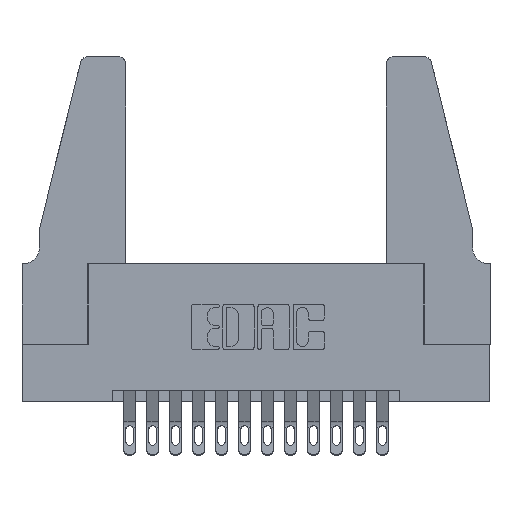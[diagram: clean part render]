
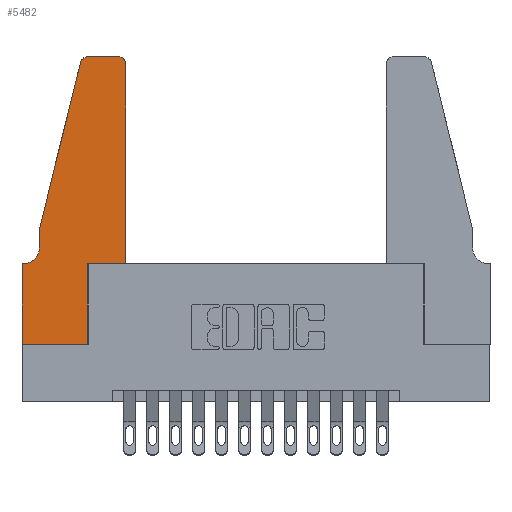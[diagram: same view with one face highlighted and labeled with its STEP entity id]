
A CAD part, top view. The second image highlights one B-rep face of the part: STEP entity #5482.
In plain terms, the highlighted planar face has unit normal (0, 0, 1).
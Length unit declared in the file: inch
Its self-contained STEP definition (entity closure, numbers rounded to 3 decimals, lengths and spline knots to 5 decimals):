
#66 = DIRECTION ( 'NONE',  ( 1., 0., 0. ) ) ;
#68 = EDGE_CURVE ( 'NONE', #10396, #11256, #2403, .T. ) ;
#447 = ORIENTED_EDGE ( 'NONE', *, *, #14626, .T. ) ;
#499 = DIRECTION ( 'NONE',  ( 1., 0., 0. ) ) ;
#636 = ORIENTED_EDGE ( 'NONE', *, *, #12247, .T. ) ;
#896 = DIRECTION ( 'NONE',  ( -1., 0., 0. ) ) ;
#1134 = VECTOR ( 'NONE', #2649, 39.37008 ) ;
#1259 = CARTESIAN_POINT ( 'NONE',  ( 0.284, 1.25, 0.37 ) ) ;
#1602 = CIRCLE ( 'NONE', #11623, 0.03 ) ;
#1690 = CARTESIAN_POINT ( 'NONE',  ( 0., 0., 0.37 ) ) ;
#1695 = DIRECTION ( 'NONE',  ( 0., 0., -1. ) ) ;
#1731 = ORIENTED_EDGE ( 'NONE', *, *, #14459, .T. ) ;
#1764 = CARTESIAN_POINT ( 'NONE',  ( 0., 0., 0.37 ) ) ;
#2403 = CIRCLE ( 'NONE', #11865, 0.07 ) ;
#2626 = LINE ( 'NONE', #1690, #5271 ) ;
#2649 = DIRECTION ( 'NONE',  ( 0., -1., 0. ) ) ;
#2809 = VECTOR ( 'NONE', #12594, 39.37008 ) ;
#2885 = CARTESIAN_POINT ( 'NONE',  ( 0.0055, 0.42, 0.37 ) ) ;
#2941 = DIRECTION ( 'NONE',  ( 0., 0., 1. ) ) ;
#3210 = DIRECTION ( 'NONE',  ( 1., 0., 0. ) ) ;
#3845 = VECTOR ( 'NONE', #13392, 39.37008 ) ;
#4041 = LINE ( 'NONE', #14674, #3845 ) ;
#4097 = EDGE_CURVE ( 'NONE', #15137, #5922, #13738, .T. ) ;
#4309 = VERTEX_POINT ( 'NONE', #12891 ) ;
#4357 = ORIENTED_EDGE ( 'NONE', *, *, #68, .T. ) ;
#4721 = CARTESIAN_POINT ( 'NONE',  ( 0.0755, 0.5, 0.37 ) ) ;
#4800 = FACE_OUTER_BOUND ( 'NONE', #14989, .T. ) ;
#4968 = ORIENTED_EDGE ( 'NONE', *, *, #10541, .T. ) ;
#5118 = DIRECTION ( 'NONE',  ( 1., 0., 0. ) ) ;
#5167 = CARTESIAN_POINT ( 'NONE',  ( 0.4505, 0.35, 0.37 ) ) ;
#5209 = ORIENTED_EDGE ( 'NONE', *, *, #5463, .T. ) ;
#5271 = VECTOR ( 'NONE', #499, 39.37008 ) ;
#5394 = DIRECTION ( 'NONE',  ( 0., 0., 1. ) ) ;
#5406 = VECTOR ( 'NONE', #5118, 39.37008 ) ;
#5433 = VERTEX_POINT ( 'NONE', #14991 ) ;
#5463 = EDGE_CURVE ( 'NONE', #6011, #7931, #13509, .T. ) ;
#5482 = ADVANCED_FACE ( 'NONE', ( #4800 ), #13869, .T. ) ;
#5524 = VERTEX_POINT ( 'NONE', #1764 ) ;
#5792 = EDGE_CURVE ( 'NONE', #5933, #8290, #8317, .T. ) ;
#5863 = LINE ( 'NONE', #11382, #2809 ) ;
#5922 = VERTEX_POINT ( 'NONE', #4721 ) ;
#5933 = VERTEX_POINT ( 'NONE', #14878 ) ;
#6011 = VERTEX_POINT ( 'NONE', #8871 ) ;
#6137 = ORIENTED_EDGE ( 'NONE', *, *, #12800, .T. ) ;
#6397 = CARTESIAN_POINT ( 'NONE',  ( 0., 0., 0.37 ) ) ;
#6466 = CARTESIAN_POINT ( 'NONE',  ( 0.4505, 1.22, 0.37 ) ) ;
#6483 = DIRECTION ( 'NONE',  ( 0., 0., 1. ) ) ;
#6576 = VECTOR ( 'NONE', #896, 39.37008 ) ;
#7133 = EDGE_CURVE ( 'NONE', #8290, #15137, #9438, .T. ) ;
#7333 = DIRECTION ( 'NONE',  ( -1., 0., 0. ) ) ;
#7451 = AXIS2_PLACEMENT_3D ( 'NONE', #12801, #5394, #3210 ) ;
#7464 = CARTESIAN_POINT ( 'NONE',  ( 0., 0.35, 0.37 ) ) ;
#7497 = AXIS2_PLACEMENT_3D ( 'NONE', #7464, #6483, #66 ) ;
#7774 = DIRECTION ( 'NONE',  ( 1., 0., 0. ) ) ;
#7825 = CARTESIAN_POINT ( 'NONE',  ( 0.4205, 1.22, 0.37 ) ) ;
#7931 = VERTEX_POINT ( 'NONE', #10380 ) ;
#7994 = VECTOR ( 'NONE', #14859, 39.37008 ) ;
#8289 = CARTESIAN_POINT ( 'NONE',  ( 0.2605, 1.25, 0.37 ) ) ;
#8290 = VERTEX_POINT ( 'NONE', #1259 ) ;
#8317 = LINE ( 'NONE', #8289, #6576 ) ;
#8871 = CARTESIAN_POINT ( 'NONE',  ( 0.2865, 0.35, 0.37 ) ) ;
#9134 = EDGE_CURVE ( 'NONE', #5922, #10396, #11413, .T. ) ;
#9281 = CARTESIAN_POINT ( 'NONE',  ( 0.25487, 1.22718, 0.37 ) ) ;
#9438 = CIRCLE ( 'NONE', #7451, 0.03 ) ;
#9605 = ORIENTED_EDGE ( 'NONE', *, *, #7133, .T. ) ;
#9710 = VECTOR ( 'NONE', #11452, 39.37008 ) ;
#9834 = EDGE_CURVE ( 'NONE', #14442, #5933, #1602, .T. ) ;
#10009 = ORIENTED_EDGE ( 'NONE', *, *, #4097, .T. ) ;
#10142 = CARTESIAN_POINT ( 'NONE',  ( 0.0755, 0.42, 0.37 ) ) ;
#10380 = CARTESIAN_POINT ( 'NONE',  ( 0.4505, 0.35, 0.37 ) ) ;
#10396 = VERTEX_POINT ( 'NONE', #10142 ) ;
#10541 = EDGE_CURVE ( 'NONE', #4309, #6011, #4041, .T. ) ;
#11141 = CARTESIAN_POINT ( 'NONE',  ( 0.0055, 0.35, 0.37 ) ) ;
#11239 = ORIENTED_EDGE ( 'NONE', *, *, #9834, .T. ) ;
#11256 = VERTEX_POINT ( 'NONE', #11141 ) ;
#11382 = CARTESIAN_POINT ( 'NONE',  ( 0.4505, 0.35, 0.37 ) ) ;
#11413 = LINE ( 'NONE', #13669, #7994 ) ;
#11452 = DIRECTION ( 'NONE',  ( -0.239, -0.971, 0. ) ) ;
#11537 = DIRECTION ( 'NONE',  ( -1., 0., 0. ) ) ;
#11623 = AXIS2_PLACEMENT_3D ( 'NONE', #7825, #2941, #7774 ) ;
#11865 = AXIS2_PLACEMENT_3D ( 'NONE', #2885, #1695, #11537 ) ;
#12247 = EDGE_CURVE ( 'NONE', #5433, #5524, #15206, .T. ) ;
#12286 = VECTOR ( 'NONE', #7333, 39.37008 ) ;
#12594 = DIRECTION ( 'NONE',  ( 0., 1., 0. ) ) ;
#12800 = EDGE_CURVE ( 'NONE', #11256, #5433, #14064, .T. ) ;
#12801 = CARTESIAN_POINT ( 'NONE',  ( 0.284, 1.22, 0.37 ) ) ;
#12891 = CARTESIAN_POINT ( 'NONE',  ( 0.2865, 0., 0.37 ) ) ;
#13392 = DIRECTION ( 'NONE',  ( 0., 1., 0. ) ) ;
#13479 = ORIENTED_EDGE ( 'NONE', *, *, #9134, .T. ) ;
#13509 = LINE ( 'NONE', #5167, #5406 ) ;
#13669 = CARTESIAN_POINT ( 'NONE',  ( 0.0755, 0.5, 0.37 ) ) ;
#13690 = CARTESIAN_POINT ( 'NONE',  ( 0.0755, 0.5, 0.37 ) ) ;
#13738 = LINE ( 'NONE', #13690, #9710 ) ;
#13869 = PLANE ( 'NONE',  #7497 ) ;
#14064 = LINE ( 'NONE', #14158, #12286 ) ;
#14131 = ORIENTED_EDGE ( 'NONE', *, *, #5792, .T. ) ;
#14158 = CARTESIAN_POINT ( 'NONE',  ( 0.0755, 0.35, 0.37 ) ) ;
#14442 = VERTEX_POINT ( 'NONE', #6466 ) ;
#14459 = EDGE_CURVE ( 'NONE', #7931, #14442, #5863, .T. ) ;
#14626 = EDGE_CURVE ( 'NONE', #5524, #4309, #2626, .T. ) ;
#14674 = CARTESIAN_POINT ( 'NONE',  ( 0.2865, 0.35, 0.37 ) ) ;
#14859 = DIRECTION ( 'NONE',  ( 0., -1., 0. ) ) ;
#14878 = CARTESIAN_POINT ( 'NONE',  ( 0.4205, 1.25, 0.37 ) ) ;
#14989 = EDGE_LOOP ( 'NONE', ( #14131, #9605, #10009, #13479, #4357, #6137, #636, #447, #4968, #5209, #1731, #11239 ) ) ;
#14991 = CARTESIAN_POINT ( 'NONE',  ( 0., 0.35, 0.37 ) ) ;
#15137 = VERTEX_POINT ( 'NONE', #9281 ) ;
#15206 = LINE ( 'NONE', #6397, #1134 ) ;
